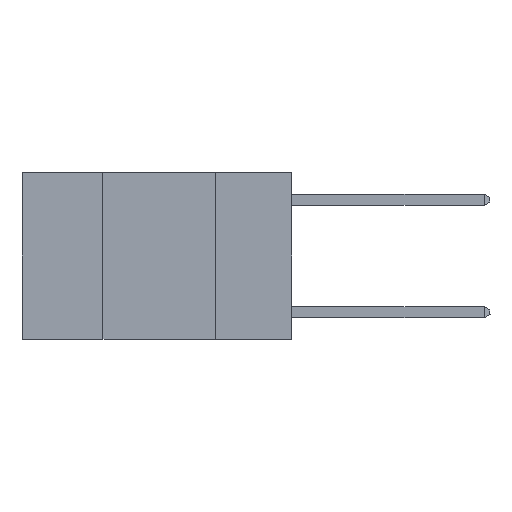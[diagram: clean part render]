
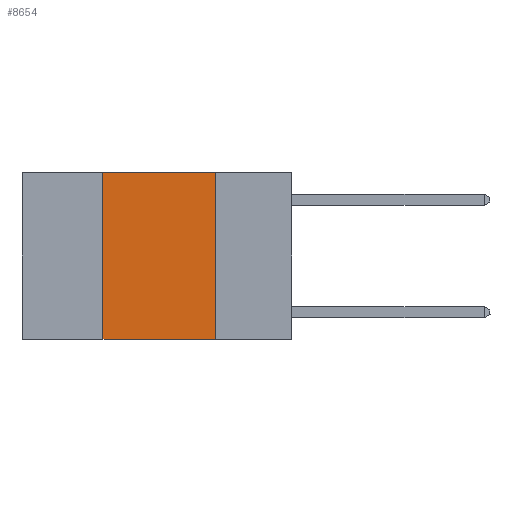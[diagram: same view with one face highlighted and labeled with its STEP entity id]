
A CAD part, left-side view. The second image highlights one B-rep face of the part: STEP entity #8654.
In plain terms, the highlighted planar face has unit normal (-1, 0, 0).
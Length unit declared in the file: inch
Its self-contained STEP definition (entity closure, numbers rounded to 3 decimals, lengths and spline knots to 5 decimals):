
#130 = LINE ( 'NONE', #9017, #5596 ) ;
#371 = AXIS2_PLACEMENT_3D ( 'NONE', #11302, #12269, #6119 ) ;
#1551 = CARTESIAN_POINT ( 'NONE',  ( 0., 0.42, 0. ) ) ;
#2325 = LINE ( 'NONE', #10865, #13036 ) ;
#2445 = VERTEX_POINT ( 'NONE', #3738 ) ;
#2957 = CARTESIAN_POINT ( 'NONE',  ( 0., 0.17, -0.37 ) ) ;
#3738 = CARTESIAN_POINT ( 'NONE',  ( 0., 0.17, 0. ) ) ;
#3820 = ORIENTED_EDGE ( 'NONE', *, *, #6307, .F. ) ;
#4842 = CARTESIAN_POINT ( 'NONE',  ( 0., 0.42, -0.37 ) ) ;
#5596 = VECTOR ( 'NONE', #10974, 39.37008 ) ;
#6119 = DIRECTION ( 'NONE',  ( 0., 0., -1. ) ) ;
#6307 = EDGE_CURVE ( 'NONE', #9188, #2445, #2325, .T. ) ;
#6444 = ORIENTED_EDGE ( 'NONE', *, *, #11114, .F. ) ;
#6883 = VERTEX_POINT ( 'NONE', #2957 ) ;
#7190 = DIRECTION ( 'NONE',  ( 0., -1., 0. ) ) ;
#7561 = LINE ( 'NONE', #10312, #12533 ) ;
#7812 = DIRECTION ( 'NONE',  ( 0., -1., 0. ) ) ;
#8282 = CARTESIAN_POINT ( 'NONE',  ( 0., 0.42, 0. ) ) ;
#8445 = EDGE_CURVE ( 'NONE', #2445, #6883, #130, .T. ) ;
#8654 = ADVANCED_FACE ( 'NONE', ( #9056 ), #10344, .F. ) ;
#9017 = CARTESIAN_POINT ( 'NONE',  ( 0., 0.17, 0. ) ) ;
#9056 = FACE_OUTER_BOUND ( 'NONE', #11736, .T. ) ;
#9180 = VECTOR ( 'NONE', #12071, 39.37008 ) ;
#9188 = VERTEX_POINT ( 'NONE', #8282 ) ;
#9801 = EDGE_CURVE ( 'NONE', #10422, #6883, #7561, .T. ) ;
#10312 = CARTESIAN_POINT ( 'NONE',  ( 0., 0.6, -0.37 ) ) ;
#10344 = PLANE ( 'NONE',  #371 ) ;
#10422 = VERTEX_POINT ( 'NONE', #4842 ) ;
#10865 = CARTESIAN_POINT ( 'NONE',  ( 0., 0.6, 0. ) ) ;
#10974 = DIRECTION ( 'NONE',  ( 0., 0., -1. ) ) ;
#11114 = EDGE_CURVE ( 'NONE', #10422, #9188, #11748, .T. ) ;
#11302 = CARTESIAN_POINT ( 'NONE',  ( 0., 0.6, 0. ) ) ;
#11507 = ORIENTED_EDGE ( 'NONE', *, *, #9801, .T. ) ;
#11736 = EDGE_LOOP ( 'NONE', ( #12193, #3820, #6444, #11507 ) ) ;
#11748 = LINE ( 'NONE', #1551, #9180 ) ;
#12071 = DIRECTION ( 'NONE',  ( 0., 0., 1. ) ) ;
#12193 = ORIENTED_EDGE ( 'NONE', *, *, #8445, .F. ) ;
#12269 = DIRECTION ( 'NONE',  ( 1., 0., 0. ) ) ;
#12533 = VECTOR ( 'NONE', #7190, 39.37008 ) ;
#13036 = VECTOR ( 'NONE', #7812, 39.37008 ) ;
